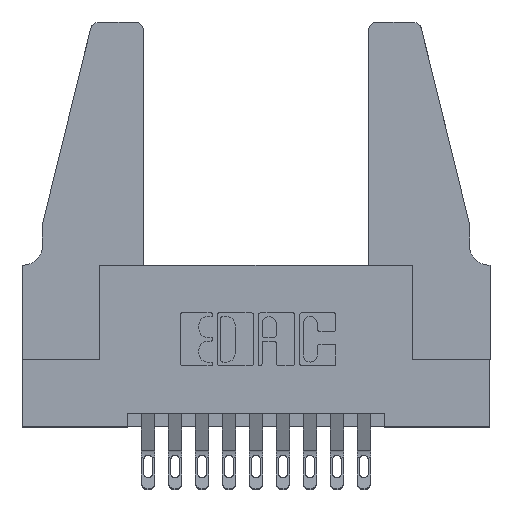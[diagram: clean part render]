
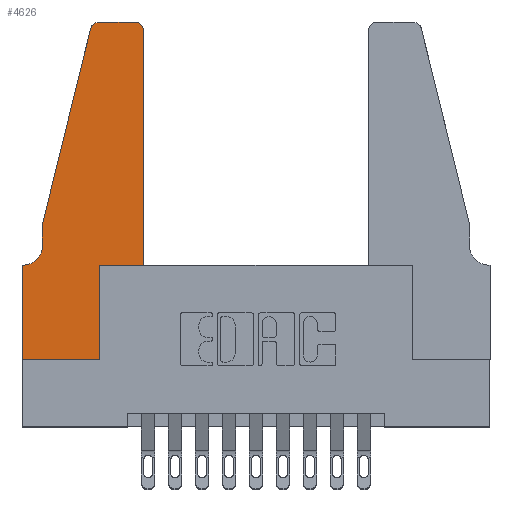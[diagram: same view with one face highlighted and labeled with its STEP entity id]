
A CAD part, top view. The second image highlights one B-rep face of the part: STEP entity #4626.
In plain terms, the highlighted planar face has unit normal (0, 0, 1).
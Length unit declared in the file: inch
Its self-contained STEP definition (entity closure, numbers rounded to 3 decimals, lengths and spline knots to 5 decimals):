
#39 = LINE ( 'NONE', #278, #809 ) ;
#99 = EDGE_CURVE ( 'NONE', #13867, #13334, #6606, .T. ) ;
#181 = DIRECTION ( 'NONE',  ( -1., 0., 0. ) ) ;
#255 = ORIENTED_EDGE ( 'NONE', *, *, #3352, .T. ) ;
#278 = CARTESIAN_POINT ( 'NONE',  ( 0., 0., 0.37 ) ) ;
#365 = EDGE_LOOP ( 'NONE', ( #5321, #8134, #8455, #11162, #8782, #255, #634, #3770, #9404, #12176, #994, #4478 ) ) ;
#580 = VERTEX_POINT ( 'NONE', #12047 ) ;
#634 = ORIENTED_EDGE ( 'NONE', *, *, #11153, .T. ) ;
#651 = LINE ( 'NONE', #692, #11856 ) ;
#679 = LINE ( 'NONE', #2667, #11873 ) ;
#692 = CARTESIAN_POINT ( 'NONE',  ( 0.4505, 0.35, 0.37 ) ) ;
#809 = VECTOR ( 'NONE', #1493, 39.37008 ) ;
#994 = ORIENTED_EDGE ( 'NONE', *, *, #9549, .T. ) ;
#1042 = VERTEX_POINT ( 'NONE', #7081 ) ;
#1160 = VECTOR ( 'NONE', #9321, 39.37008 ) ;
#1305 = CARTESIAN_POINT ( 'NONE',  ( 0.0755, 0.42, 0.37 ) ) ;
#1318 = CARTESIAN_POINT ( 'NONE',  ( 0.4205, 1.22, 0.37 ) ) ;
#1493 = DIRECTION ( 'NONE',  ( 0., -1., 0. ) ) ;
#1596 = CARTESIAN_POINT ( 'NONE',  ( 0., 0.35, 0.37 ) ) ;
#2431 = CARTESIAN_POINT ( 'NONE',  ( 0., 0., 0.37 ) ) ;
#2530 = DIRECTION ( 'NONE',  ( 1., 0., 0. ) ) ;
#2667 = CARTESIAN_POINT ( 'NONE',  ( 0.4505, 0.35, 0.37 ) ) ;
#3255 = CARTESIAN_POINT ( 'NONE',  ( 0.0755, 0.35, 0.37 ) ) ;
#3352 = EDGE_CURVE ( 'NONE', #7763, #10174, #6360, .T. ) ;
#3455 = VECTOR ( 'NONE', #4385, 39.37008 ) ;
#3537 = EDGE_CURVE ( 'NONE', #11064, #10365, #7161, .T. ) ;
#3770 = ORIENTED_EDGE ( 'NONE', *, *, #3537, .T. ) ;
#3793 = EDGE_CURVE ( 'NONE', #8441, #580, #651, .T. ) ;
#4385 = DIRECTION ( 'NONE',  ( -1., 0., 0. ) ) ;
#4478 = ORIENTED_EDGE ( 'NONE', *, *, #11614, .T. ) ;
#4620 = CARTESIAN_POINT ( 'NONE',  ( 0.0755, 0.5, 0.37 ) ) ;
#4626 = ADVANCED_FACE ( 'NONE', ( #13773 ), #11905, .T. ) ;
#4931 = AXIS2_PLACEMENT_3D ( 'NONE', #1318, #8994, #2530 ) ;
#5223 = VECTOR ( 'NONE', #7183, 39.37008 ) ;
#5282 = VERTEX_POINT ( 'NONE', #4620 ) ;
#5321 = ORIENTED_EDGE ( 'NONE', *, *, #13104, .T. ) ;
#5361 = EDGE_CURVE ( 'NONE', #5282, #12287, #9537, .T. ) ;
#5492 = CARTESIAN_POINT ( 'NONE',  ( 0.0755, 0.5, 0.37 ) ) ;
#5570 = LINE ( 'NONE', #5492, #13225 ) ;
#5676 = DIRECTION ( 'NONE',  ( 0., 0., 1. ) ) ;
#5790 = EDGE_CURVE ( 'NONE', #12287, #7763, #10162, .T. ) ;
#6011 = DIRECTION ( 'NONE',  ( 0., 1., 0. ) ) ;
#6184 = CARTESIAN_POINT ( 'NONE',  ( 0.2865, 0.35, 0.37 ) ) ;
#6360 = LINE ( 'NONE', #3255, #3455 ) ;
#6606 = CIRCLE ( 'NONE', #12549, 0.03 ) ;
#6959 = DIRECTION ( 'NONE',  ( 0., 0., -1. ) ) ;
#7081 = CARTESIAN_POINT ( 'NONE',  ( 0.4205, 1.25, 0.37 ) ) ;
#7161 = LINE ( 'NONE', #2431, #12033 ) ;
#7183 = DIRECTION ( 'NONE',  ( -1., 0., 0. ) ) ;
#7568 = CIRCLE ( 'NONE', #4931, 0.03 ) ;
#7763 = VERTEX_POINT ( 'NONE', #9264 ) ;
#7985 = VECTOR ( 'NONE', #10638, 39.37008 ) ;
#8025 = LINE ( 'NONE', #11285, #5223 ) ;
#8134 = ORIENTED_EDGE ( 'NONE', *, *, #99, .T. ) ;
#8239 = CARTESIAN_POINT ( 'NONE',  ( 0.4505, 1.22, 0.37 ) ) ;
#8305 = CARTESIAN_POINT ( 'NONE',  ( 0.0755, 0.5, 0.37 ) ) ;
#8441 = VERTEX_POINT ( 'NONE', #6184 ) ;
#8455 = ORIENTED_EDGE ( 'NONE', *, *, #12701, .T. ) ;
#8782 = ORIENTED_EDGE ( 'NONE', *, *, #5790, .T. ) ;
#8994 = DIRECTION ( 'NONE',  ( 0., 0., 1. ) ) ;
#9220 = EDGE_CURVE ( 'NONE', #10365, #8441, #10713, .T. ) ;
#9264 = CARTESIAN_POINT ( 'NONE',  ( 0.0055, 0.35, 0.37 ) ) ;
#9268 = AXIS2_PLACEMENT_3D ( 'NONE', #13175, #6959, #181 ) ;
#9321 = DIRECTION ( 'NONE',  ( 0., -1., 0. ) ) ;
#9404 = ORIENTED_EDGE ( 'NONE', *, *, #9220, .T. ) ;
#9436 = DIRECTION ( 'NONE',  ( 1., 0., 0. ) ) ;
#9470 = DIRECTION ( 'NONE',  ( 1., 0., 0. ) ) ;
#9537 = LINE ( 'NONE', #8305, #1160 ) ;
#9549 = EDGE_CURVE ( 'NONE', #580, #11761, #679, .T. ) ;
#9614 = CARTESIAN_POINT ( 'NONE',  ( 0.284, 1.22, 0.37 ) ) ;
#10162 = CIRCLE ( 'NONE', #9268, 0.07 ) ;
#10174 = VERTEX_POINT ( 'NONE', #1596 ) ;
#10365 = VERTEX_POINT ( 'NONE', #11566 ) ;
#10638 = DIRECTION ( 'NONE',  ( 0., 1., 0. ) ) ;
#10713 = LINE ( 'NONE', #11646, #7985 ) ;
#10840 = CARTESIAN_POINT ( 'NONE',  ( 0., 0.35, 0.37 ) ) ;
#10954 = DIRECTION ( 'NONE',  ( 1., 0., 0. ) ) ;
#10966 = AXIS2_PLACEMENT_3D ( 'NONE', #10840, #5676, #12974 ) ;
#11064 = VERTEX_POINT ( 'NONE', #12133 ) ;
#11153 = EDGE_CURVE ( 'NONE', #10174, #11064, #39, .T. ) ;
#11162 = ORIENTED_EDGE ( 'NONE', *, *, #5361, .T. ) ;
#11285 = CARTESIAN_POINT ( 'NONE',  ( 0.2605, 1.25, 0.37 ) ) ;
#11566 = CARTESIAN_POINT ( 'NONE',  ( 0.2865, 0., 0.37 ) ) ;
#11614 = EDGE_CURVE ( 'NONE', #11761, #1042, #7568, .T. ) ;
#11639 = CARTESIAN_POINT ( 'NONE',  ( 0.284, 1.25, 0.37 ) ) ;
#11646 = CARTESIAN_POINT ( 'NONE',  ( 0.2865, 0.35, 0.37 ) ) ;
#11714 = DIRECTION ( 'NONE',  ( -0.239, -0.971, 0. ) ) ;
#11745 = CARTESIAN_POINT ( 'NONE',  ( 0.25487, 1.22718, 0.37 ) ) ;
#11761 = VERTEX_POINT ( 'NONE', #8239 ) ;
#11856 = VECTOR ( 'NONE', #9470, 39.37008 ) ;
#11873 = VECTOR ( 'NONE', #6011, 39.37008 ) ;
#11905 = PLANE ( 'NONE',  #10966 ) ;
#12033 = VECTOR ( 'NONE', #10954, 39.37008 ) ;
#12047 = CARTESIAN_POINT ( 'NONE',  ( 0.4505, 0.35, 0.37 ) ) ;
#12133 = CARTESIAN_POINT ( 'NONE',  ( 0., 0., 0.37 ) ) ;
#12176 = ORIENTED_EDGE ( 'NONE', *, *, #3793, .T. ) ;
#12287 = VERTEX_POINT ( 'NONE', #1305 ) ;
#12549 = AXIS2_PLACEMENT_3D ( 'NONE', #9614, #13611, #9436 ) ;
#12701 = EDGE_CURVE ( 'NONE', #13334, #5282, #5570, .T. ) ;
#12974 = DIRECTION ( 'NONE',  ( 1., 0., 0. ) ) ;
#13104 = EDGE_CURVE ( 'NONE', #1042, #13867, #8025, .T. ) ;
#13175 = CARTESIAN_POINT ( 'NONE',  ( 0.0055, 0.42, 0.37 ) ) ;
#13225 = VECTOR ( 'NONE', #11714, 39.37008 ) ;
#13334 = VERTEX_POINT ( 'NONE', #11745 ) ;
#13611 = DIRECTION ( 'NONE',  ( 0., 0., 1. ) ) ;
#13773 = FACE_OUTER_BOUND ( 'NONE', #365, .T. ) ;
#13867 = VERTEX_POINT ( 'NONE', #11639 ) ;
